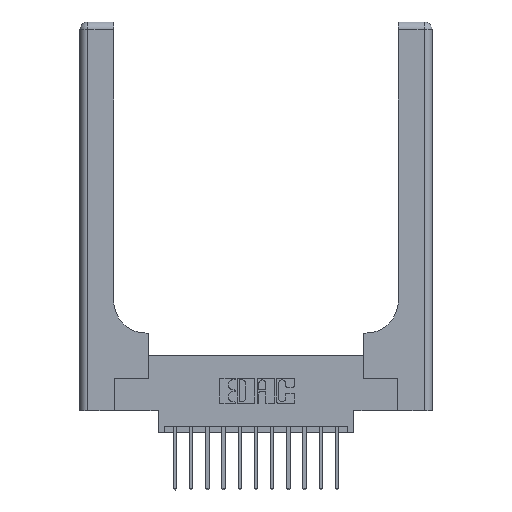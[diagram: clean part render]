
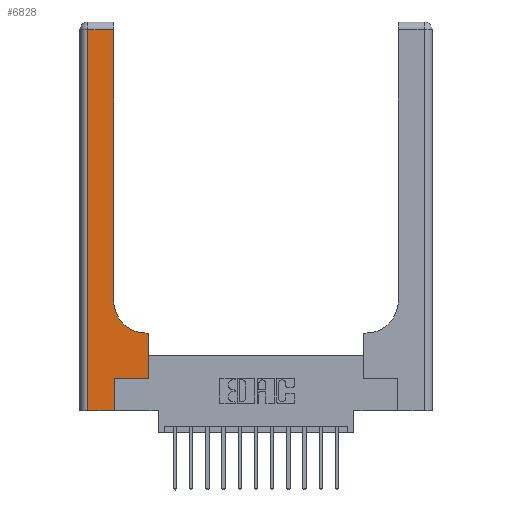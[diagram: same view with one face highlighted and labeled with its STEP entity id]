
A CAD part, top view. The second image highlights one B-rep face of the part: STEP entity #6828.
In plain terms, the highlighted planar face has unit normal (0, 0, 1).
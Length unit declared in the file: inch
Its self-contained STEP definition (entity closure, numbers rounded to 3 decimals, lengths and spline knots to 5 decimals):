
#558 = VECTOR ( 'NONE', #8157, 39.37008 ) ;
#588 = ORIENTED_EDGE ( 'NONE', *, *, #10510, .T. ) ;
#655 = LINE ( 'NONE', #8044, #7540 ) ;
#1249 = DIRECTION ( 'NONE',  ( 0., 1., 0. ) ) ;
#1708 = VECTOR ( 'NONE', #13051, 39.37008 ) ;
#1725 = VECTOR ( 'NONE', #5570, 39.37008 ) ;
#1781 = CARTESIAN_POINT ( 'NONE',  ( 0.06, 0., 0.37 ) ) ;
#1819 = EDGE_CURVE ( 'NONE', #7101, #10125, #4100, .T. ) ;
#1841 = PLANE ( 'NONE',  #9276 ) ;
#2334 = ORIENTED_EDGE ( 'NONE', *, *, #10052, .T. ) ;
#2596 = LINE ( 'NONE', #2692, #16297 ) ;
#2692 = CARTESIAN_POINT ( 'NONE',  ( 0.528, 0.25, 0.37 ) ) ;
#3098 = EDGE_CURVE ( 'NONE', #13287, #7628, #655, .T. ) ;
#3136 = CARTESIAN_POINT ( 'NONE',  ( 0., 3., 0.37 ) ) ;
#3285 = CARTESIAN_POINT ( 'NONE',  ( 0.26, 0.85, 0.37 ) ) ;
#3351 = FACE_OUTER_BOUND ( 'NONE', #5332, .T. ) ;
#3546 = DIRECTION ( 'NONE',  ( 1., 0., 0. ) ) ;
#3646 = VERTEX_POINT ( 'NONE', #1781 ) ;
#3689 = CARTESIAN_POINT ( 'NONE',  ( 0.06, 2.94, 0.37 ) ) ;
#3711 = VECTOR ( 'NONE', #5273, 39.37008 ) ;
#3961 = CARTESIAN_POINT ( 'NONE',  ( 0., 0., 0.37 ) ) ;
#3967 = VERTEX_POINT ( 'NONE', #3689 ) ;
#4015 = CARTESIAN_POINT ( 'NONE',  ( 0.26, 3., 0.37 ) ) ;
#4100 = LINE ( 'NONE', #8989, #10953 ) ;
#4444 = DIRECTION ( 'NONE',  ( 0., 0., -1. ) ) ;
#4465 = ORIENTED_EDGE ( 'NONE', *, *, #1819, .T. ) ;
#4609 = DIRECTION ( 'NONE',  ( 0., 0., -1. ) ) ;
#4828 = VERTEX_POINT ( 'NONE', #11905 ) ;
#5273 = DIRECTION ( 'NONE',  ( 1., 0., 0. ) ) ;
#5332 = EDGE_LOOP ( 'NONE', ( #588, #2334, #9979, #11001, #4465, #7476, #13185, #15958, #15275 ) ) ;
#5358 = EDGE_CURVE ( 'NONE', #14675, #13287, #2596, .T. ) ;
#5570 = DIRECTION ( 'NONE',  ( -1., 0., 0. ) ) ;
#6150 = LINE ( 'NONE', #12580, #16430 ) ;
#6156 = CARTESIAN_POINT ( 'NONE',  ( 0.51, 0.6, 0.37 ) ) ;
#6828 = ADVANCED_FACE ( 'NONE', ( #3351 ), #1841, .F. ) ;
#6912 = EDGE_CURVE ( 'NONE', #7628, #10201, #12033, .T. ) ;
#7101 = VERTEX_POINT ( 'NONE', #12674 ) ;
#7476 = ORIENTED_EDGE ( 'NONE', *, *, #10942, .T. ) ;
#7540 = VECTOR ( 'NONE', #11900, 39.37008 ) ;
#7628 = VERTEX_POINT ( 'NONE', #6156 ) ;
#8044 = CARTESIAN_POINT ( 'NONE',  ( 0.26, 0.6, 0.37 ) ) ;
#8157 = DIRECTION ( 'NONE',  ( 0., -1., 0. ) ) ;
#8656 = EDGE_CURVE ( 'NONE', #3967, #3646, #10834, .T. ) ;
#8989 = CARTESIAN_POINT ( 'NONE',  ( 0.265, 0., 0.37 ) ) ;
#9126 = DIRECTION ( 'NONE',  ( 0., 1., 0. ) ) ;
#9157 = CARTESIAN_POINT ( 'NONE',  ( 0.528, 0.6, 0.37 ) ) ;
#9276 = AXIS2_PLACEMENT_3D ( 'NONE', #3136, #4444, #13466 ) ;
#9442 = CARTESIAN_POINT ( 'NONE',  ( 0.06, 3., 0.37 ) ) ;
#9979 = ORIENTED_EDGE ( 'NONE', *, *, #8656, .T. ) ;
#10052 = EDGE_CURVE ( 'NONE', #4828, #3967, #12010, .T. ) ;
#10125 = VERTEX_POINT ( 'NONE', #16031 ) ;
#10201 = VERTEX_POINT ( 'NONE', #3285 ) ;
#10329 = CARTESIAN_POINT ( 'NONE',  ( 0.528, 0.25, 0.37 ) ) ;
#10510 = EDGE_CURVE ( 'NONE', #10201, #4828, #11591, .T. ) ;
#10572 = LINE ( 'NONE', #3961, #3711 ) ;
#10834 = LINE ( 'NONE', #9442, #558 ) ;
#10942 = EDGE_CURVE ( 'NONE', #10125, #14675, #6150, .T. ) ;
#10953 = VECTOR ( 'NONE', #1249, 39.37008 ) ;
#11001 = ORIENTED_EDGE ( 'NONE', *, *, #11551, .T. ) ;
#11551 = EDGE_CURVE ( 'NONE', #3646, #7101, #10572, .T. ) ;
#11591 = LINE ( 'NONE', #4015, #1708 ) ;
#11859 = AXIS2_PLACEMENT_3D ( 'NONE', #12330, #4609, #13642 ) ;
#11900 = DIRECTION ( 'NONE',  ( -1., 0., 0. ) ) ;
#11905 = CARTESIAN_POINT ( 'NONE',  ( 0.26, 2.94, 0.37 ) ) ;
#12010 = LINE ( 'NONE', #14574, #1725 ) ;
#12033 = CIRCLE ( 'NONE', #11859, 0.25 ) ;
#12330 = CARTESIAN_POINT ( 'NONE',  ( 0.51, 0.85, 0.37 ) ) ;
#12580 = CARTESIAN_POINT ( 'NONE',  ( 0.265, 0.25, 0.37 ) ) ;
#12674 = CARTESIAN_POINT ( 'NONE',  ( 0.265, 0., 0.37 ) ) ;
#13051 = DIRECTION ( 'NONE',  ( 0., 1., 0. ) ) ;
#13185 = ORIENTED_EDGE ( 'NONE', *, *, #5358, .T. ) ;
#13287 = VERTEX_POINT ( 'NONE', #9157 ) ;
#13466 = DIRECTION ( 'NONE',  ( -1., 0., 0. ) ) ;
#13642 = DIRECTION ( 'NONE',  ( 1., 0., 0. ) ) ;
#14574 = CARTESIAN_POINT ( 'NONE',  ( 0., 2.94, 0.37 ) ) ;
#14675 = VERTEX_POINT ( 'NONE', #10329 ) ;
#15275 = ORIENTED_EDGE ( 'NONE', *, *, #6912, .T. ) ;
#15958 = ORIENTED_EDGE ( 'NONE', *, *, #3098, .T. ) ;
#16031 = CARTESIAN_POINT ( 'NONE',  ( 0.265, 0.25, 0.37 ) ) ;
#16297 = VECTOR ( 'NONE', #9126, 39.37008 ) ;
#16430 = VECTOR ( 'NONE', #3546, 39.37008 ) ;
